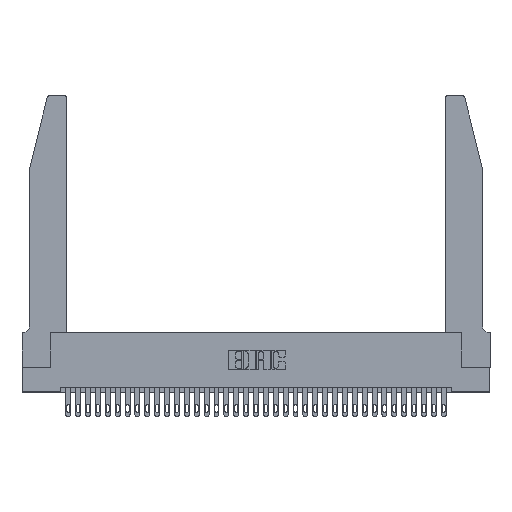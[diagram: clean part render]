
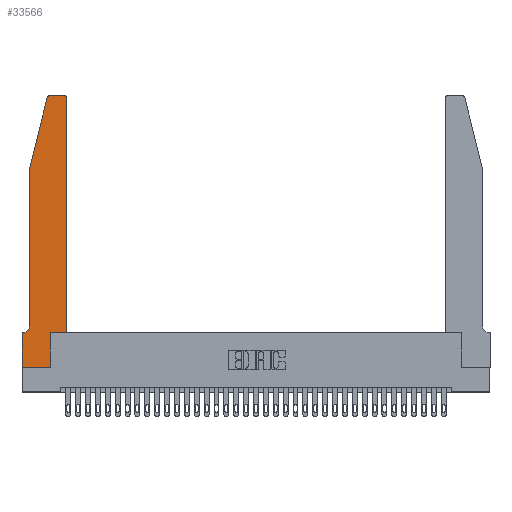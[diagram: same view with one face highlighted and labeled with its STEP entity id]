
A CAD part, top view. The second image highlights one B-rep face of the part: STEP entity #33566.
In plain terms, the highlighted planar face has unit normal (0, 0, 1).
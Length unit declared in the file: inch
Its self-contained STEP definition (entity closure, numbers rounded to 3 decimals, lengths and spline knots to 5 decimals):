
#252 = EDGE_CURVE ( 'NONE', #14294, #24534, #29818, .T. ) ;
#465 = DIRECTION ( 'NONE',  ( -1., 0., 0. ) ) ;
#1452 = VECTOR ( 'NONE', #3084, 39.37008 ) ;
#1488 = DIRECTION ( 'NONE',  ( 0., 0., 1. ) ) ;
#1683 = EDGE_CURVE ( 'NONE', #24534, #17879, #10387, .T. ) ;
#1691 = ORIENTED_EDGE ( 'NONE', *, *, #16143, .T. ) ;
#2932 = CARTESIAN_POINT ( 'NONE',  ( 0.0055, 0.35, 0.37 ) ) ;
#2965 = EDGE_LOOP ( 'NONE', ( #6270, #26282, #22747, #9221, #26839, #14363, #10615, #12459, #22111, #1691, #11001, #11572 ) ) ;
#3084 = DIRECTION ( 'NONE',  ( 0., -1., 0. ) ) ;
#3826 = EDGE_CURVE ( 'NONE', #22808, #8183, #24370, .T. ) ;
#4071 = VECTOR ( 'NONE', #18996, 39.37008 ) ;
#4759 = CARTESIAN_POINT ( 'NONE',  ( 0.284, 2.75, 0.37 ) ) ;
#4798 = DIRECTION ( 'NONE',  ( 0., 1., 0. ) ) ;
#4863 = EDGE_CURVE ( 'NONE', #17879, #5953, #11757, .T. ) ;
#5418 = CIRCLE ( 'NONE', #32816, 0.07 ) ;
#5939 = FACE_OUTER_BOUND ( 'NONE', #2965, .T. ) ;
#5953 = VERTEX_POINT ( 'NONE', #4759 ) ;
#6230 = CARTESIAN_POINT ( 'NONE',  ( 0.0055, 0.42, 0.37 ) ) ;
#6270 = ORIENTED_EDGE ( 'NONE', *, *, #4863, .T. ) ;
#6508 = DIRECTION ( 'NONE',  ( 1., 0., 0. ) ) ;
#6602 = VECTOR ( 'NONE', #465, 39.37008 ) ;
#7330 = EDGE_CURVE ( 'NONE', #8183, #25590, #29747, .T. ) ;
#7426 = CARTESIAN_POINT ( 'NONE',  ( 0.0755, 2., 0.37 ) ) ;
#8183 = VERTEX_POINT ( 'NONE', #7426 ) ;
#8491 = DIRECTION ( 'NONE',  ( 0., 0., 1. ) ) ;
#8711 = AXIS2_PLACEMENT_3D ( 'NONE', #20594, #9798, #17707 ) ;
#9009 = CARTESIAN_POINT ( 'NONE',  ( 0., 0., 0.37 ) ) ;
#9221 = ORIENTED_EDGE ( 'NONE', *, *, #7330, .T. ) ;
#9798 = DIRECTION ( 'NONE',  ( 0., 0., 1. ) ) ;
#10387 = CIRCLE ( 'NONE', #28014, 0.03 ) ;
#10615 = ORIENTED_EDGE ( 'NONE', *, *, #29620, .T. ) ;
#11001 = ORIENTED_EDGE ( 'NONE', *, *, #252, .T. ) ;
#11132 = CARTESIAN_POINT ( 'NONE',  ( 0., 0., 0.37 ) ) ;
#11572 = ORIENTED_EDGE ( 'NONE', *, *, #1683, .T. ) ;
#11757 = LINE ( 'NONE', #15880, #4071 ) ;
#12027 = EDGE_CURVE ( 'NONE', #30229, #34514, #24710, .T. ) ;
#12266 = CARTESIAN_POINT ( 'NONE',  ( 0., 0.35, 0.37 ) ) ;
#12326 = CARTESIAN_POINT ( 'NONE',  ( 0.25487, 2.72718, 0.37 ) ) ;
#12459 = ORIENTED_EDGE ( 'NONE', *, *, #22648, .T. ) ;
#13269 = CARTESIAN_POINT ( 'NONE',  ( 0.0755, 2., 0.37 ) ) ;
#13574 = VECTOR ( 'NONE', #20971, 39.37008 ) ;
#13618 = CARTESIAN_POINT ( 'NONE',  ( 0.4505, 2.72, 0.37 ) ) ;
#14022 = DIRECTION ( 'NONE',  ( 1., 0., 0. ) ) ;
#14294 = VERTEX_POINT ( 'NONE', #23131 ) ;
#14363 = ORIENTED_EDGE ( 'NONE', *, *, #12027, .T. ) ;
#14428 = CARTESIAN_POINT ( 'NONE',  ( 0.2865, 0.35, 0.37 ) ) ;
#14652 = DIRECTION ( 'NONE',  ( 0., 0., -1. ) ) ;
#14987 = CARTESIAN_POINT ( 'NONE',  ( 0.2865, 0.35, 0.37 ) ) ;
#15880 = CARTESIAN_POINT ( 'NONE',  ( 0.2605, 2.75, 0.37 ) ) ;
#16125 = LINE ( 'NONE', #11132, #1452 ) ;
#16143 = EDGE_CURVE ( 'NONE', #19739, #14294, #16451, .T. ) ;
#16451 = LINE ( 'NONE', #30906, #27595 ) ;
#16776 = CARTESIAN_POINT ( 'NONE',  ( 0., 0.35, 0.37 ) ) ;
#16905 = CARTESIAN_POINT ( 'NONE',  ( 0.4505, 0.35, 0.37 ) ) ;
#17290 = DIRECTION ( 'NONE',  ( 1., 0., 0. ) ) ;
#17694 = DIRECTION ( 'NONE',  ( 1., 0., 0. ) ) ;
#17707 = DIRECTION ( 'NONE',  ( 1., 0., 0. ) ) ;
#17879 = VERTEX_POINT ( 'NONE', #28719 ) ;
#18996 = DIRECTION ( 'NONE',  ( -1., 0., 0. ) ) ;
#19171 = AXIS2_PLACEMENT_3D ( 'NONE', #16776, #8491, #14022 ) ;
#19739 = VERTEX_POINT ( 'NONE', #14428 ) ;
#20453 = EDGE_CURVE ( 'NONE', #25590, #30229, #5418, .T. ) ;
#20594 = CARTESIAN_POINT ( 'NONE',  ( 0.284, 2.72, 0.37 ) ) ;
#20618 = LINE ( 'NONE', #9009, #34443 ) ;
#20971 = DIRECTION ( 'NONE',  ( 0., 1., 0. ) ) ;
#22111 = ORIENTED_EDGE ( 'NONE', *, *, #35683, .T. ) ;
#22251 = CARTESIAN_POINT ( 'NONE',  ( 0.0755, 0.35, 0.37 ) ) ;
#22648 = EDGE_CURVE ( 'NONE', #28457, #26869, #20618, .T. ) ;
#22747 = ORIENTED_EDGE ( 'NONE', *, *, #3826, .T. ) ;
#22754 = PLANE ( 'NONE',  #19171 ) ;
#22808 = VERTEX_POINT ( 'NONE', #12326 ) ;
#23131 = CARTESIAN_POINT ( 'NONE',  ( 0.4505, 0.35, 0.37 ) ) ;
#23529 = DIRECTION ( 'NONE',  ( -1., 0., 0. ) ) ;
#24370 = LINE ( 'NONE', #13269, #30766 ) ;
#24534 = VERTEX_POINT ( 'NONE', #13618 ) ;
#24710 = LINE ( 'NONE', #22251, #6602 ) ;
#25590 = VERTEX_POINT ( 'NONE', #35362 ) ;
#26282 = ORIENTED_EDGE ( 'NONE', *, *, #30613, .T. ) ;
#26839 = ORIENTED_EDGE ( 'NONE', *, *, #20453, .T. ) ;
#26869 = VERTEX_POINT ( 'NONE', #30385 ) ;
#27595 = VECTOR ( 'NONE', #6508, 39.37008 ) ;
#28014 = AXIS2_PLACEMENT_3D ( 'NONE', #34204, #1488, #17694 ) ;
#28042 = VECTOR ( 'NONE', #4798, 39.37008 ) ;
#28312 = DIRECTION ( 'NONE',  ( 0., -1., 0. ) ) ;
#28403 = VECTOR ( 'NONE', #28312, 39.37008 ) ;
#28457 = VERTEX_POINT ( 'NONE', #33815 ) ;
#28719 = CARTESIAN_POINT ( 'NONE',  ( 0.4205, 2.75, 0.37 ) ) ;
#29012 = LINE ( 'NONE', #14987, #13574 ) ;
#29620 = EDGE_CURVE ( 'NONE', #34514, #28457, #16125, .T. ) ;
#29747 = LINE ( 'NONE', #30624, #28403 ) ;
#29818 = LINE ( 'NONE', #16905, #28042 ) ;
#30229 = VERTEX_POINT ( 'NONE', #2932 ) ;
#30385 = CARTESIAN_POINT ( 'NONE',  ( 0.2865, 0., 0.37 ) ) ;
#30613 = EDGE_CURVE ( 'NONE', #5953, #22808, #31938, .T. ) ;
#30624 = CARTESIAN_POINT ( 'NONE',  ( 0.0755, 2., 0.37 ) ) ;
#30766 = VECTOR ( 'NONE', #35677, 39.37008 ) ;
#30906 = CARTESIAN_POINT ( 'NONE',  ( 0.4505, 0.35, 0.37 ) ) ;
#31938 = CIRCLE ( 'NONE', #8711, 0.03 ) ;
#32816 = AXIS2_PLACEMENT_3D ( 'NONE', #6230, #14652, #23529 ) ;
#33566 = ADVANCED_FACE ( 'NONE', ( #5939 ), #22754, .T. ) ;
#33815 = CARTESIAN_POINT ( 'NONE',  ( 0., 0., 0.37 ) ) ;
#34204 = CARTESIAN_POINT ( 'NONE',  ( 0.4205, 2.72, 0.37 ) ) ;
#34443 = VECTOR ( 'NONE', #17290, 39.37008 ) ;
#34514 = VERTEX_POINT ( 'NONE', #12266 ) ;
#35362 = CARTESIAN_POINT ( 'NONE',  ( 0.0755, 0.42, 0.37 ) ) ;
#35677 = DIRECTION ( 'NONE',  ( -0.239, -0.971, 0. ) ) ;
#35683 = EDGE_CURVE ( 'NONE', #26869, #19739, #29012, .T. ) ;
